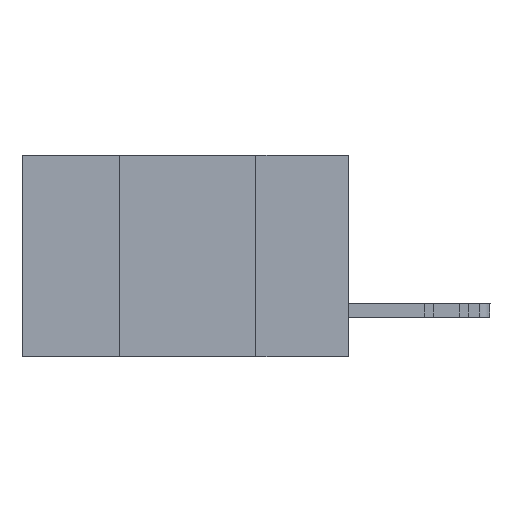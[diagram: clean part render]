
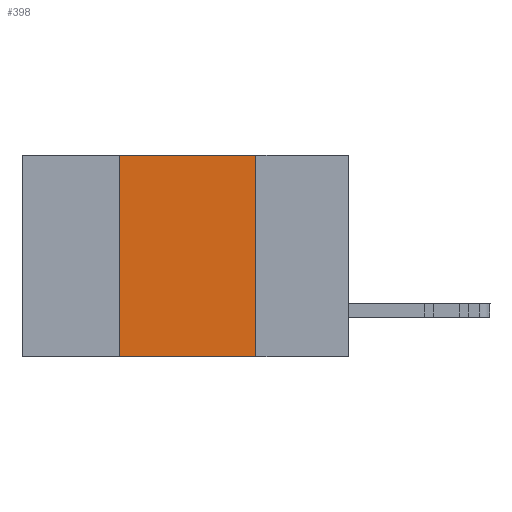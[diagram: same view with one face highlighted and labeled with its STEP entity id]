
A CAD part, left-side view. The second image highlights one B-rep face of the part: STEP entity #398.
In plain terms, the highlighted planar face has unit normal (-1, 0, 0).
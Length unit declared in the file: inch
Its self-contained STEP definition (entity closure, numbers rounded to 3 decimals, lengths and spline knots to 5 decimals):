
#398 = ADVANCED_FACE ( 'NONE', ( #12046 ), #25595, .F. ) ;
#1193 = EDGE_CURVE ( 'NONE', #23810, #17513, #17260, .T. ) ;
#1383 = CARTESIAN_POINT ( 'NONE',  ( 0., 0.42, -0.37 ) ) ;
#3088 = EDGE_CURVE ( 'NONE', #17513, #9275, #10351, .T. ) ;
#3122 = ORIENTED_EDGE ( 'NONE', *, *, #6350, .T. ) ;
#3930 = LINE ( 'NONE', #1383, #9338 ) ;
#4314 = CARTESIAN_POINT ( 'NONE',  ( 0., 0.17, -0.37 ) ) ;
#5505 = DIRECTION ( 'NONE',  ( 0., 0., 1. ) ) ;
#5763 = CARTESIAN_POINT ( 'NONE',  ( 0., 0.6, -0.37 ) ) ;
#6350 = EDGE_CURVE ( 'NONE', #22044, #9275, #11061, .T. ) ;
#6410 = DIRECTION ( 'NONE',  ( 0., 0., -1. ) ) ;
#6459 = DIRECTION ( 'NONE',  ( 1., 0., 0. ) ) ;
#7282 = VECTOR ( 'NONE', #18100, 39.37008 ) ;
#8002 = DIRECTION ( 'NONE',  ( 0., -1., 0. ) ) ;
#9275 = VERTEX_POINT ( 'NONE', #4314 ) ;
#9338 = VECTOR ( 'NONE', #5505, 39.37008 ) ;
#10351 = LINE ( 'NONE', #21816, #15680 ) ;
#10426 = VECTOR ( 'NONE', #8002, 39.37008 ) ;
#11061 = LINE ( 'NONE', #5763, #10426 ) ;
#11356 = ORIENTED_EDGE ( 'NONE', *, *, #3088, .F. ) ;
#11493 = CARTESIAN_POINT ( 'NONE',  ( 0., 0.42, 0. ) ) ;
#11651 = CARTESIAN_POINT ( 'NONE',  ( 0., 0.17, 0. ) ) ;
#11850 = CARTESIAN_POINT ( 'NONE',  ( 0., 0.42, -0.37 ) ) ;
#12046 = FACE_OUTER_BOUND ( 'NONE', #25379, .T. ) ;
#12249 = EDGE_CURVE ( 'NONE', #22044, #23810, #3930, .T. ) ;
#12622 = ORIENTED_EDGE ( 'NONE', *, *, #1193, .F. ) ;
#15680 = VECTOR ( 'NONE', #21511, 39.37008 ) ;
#17260 = LINE ( 'NONE', #18136, #7282 ) ;
#17513 = VERTEX_POINT ( 'NONE', #11651 ) ;
#18100 = DIRECTION ( 'NONE',  ( 0., -1., 0. ) ) ;
#18136 = CARTESIAN_POINT ( 'NONE',  ( 0., 0.6, 0. ) ) ;
#20592 = CARTESIAN_POINT ( 'NONE',  ( 0., 0.6, 0. ) ) ;
#21511 = DIRECTION ( 'NONE',  ( 0., 0., -1. ) ) ;
#21610 = AXIS2_PLACEMENT_3D ( 'NONE', #20592, #6459, #6410 ) ;
#21816 = CARTESIAN_POINT ( 'NONE',  ( 0., 0.17, -0.37 ) ) ;
#22044 = VERTEX_POINT ( 'NONE', #11850 ) ;
#23048 = ORIENTED_EDGE ( 'NONE', *, *, #12249, .F. ) ;
#23810 = VERTEX_POINT ( 'NONE', #11493 ) ;
#25379 = EDGE_LOOP ( 'NONE', ( #11356, #12622, #23048, #3122 ) ) ;
#25595 = PLANE ( 'NONE',  #21610 ) ;
